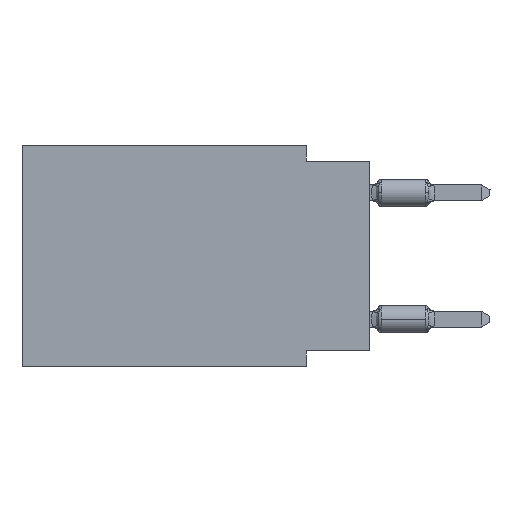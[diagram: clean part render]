
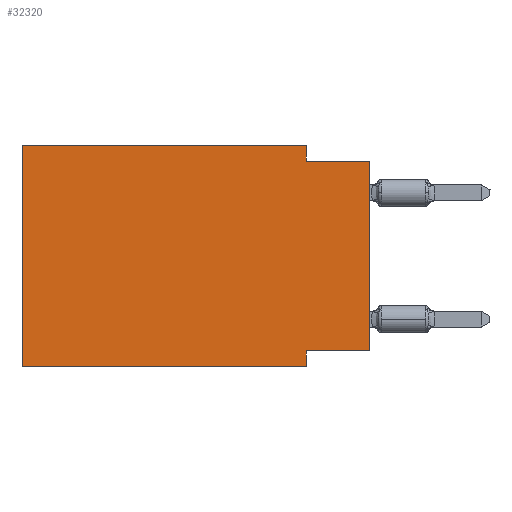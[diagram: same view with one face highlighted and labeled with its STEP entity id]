
A CAD part, left-side view. The second image highlights one B-rep face of the part: STEP entity #32320.
In plain terms, the highlighted planar face has unit normal (-1, 0, 0).
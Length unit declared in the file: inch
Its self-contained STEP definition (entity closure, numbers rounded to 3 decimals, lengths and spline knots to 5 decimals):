
#1415 = CARTESIAN_POINT ( 'NONE',  ( 0., 0., 0. ) ) ;
#2470 = ORIENTED_EDGE ( 'NONE', *, *, #6473, .T. ) ;
#2503 = DIRECTION ( 'NONE',  ( 0., 0., -1. ) ) ;
#2702 = VERTEX_POINT ( 'NONE', #35628 ) ;
#2811 = CARTESIAN_POINT ( 'NONE',  ( 0., 0.55, -0.35 ) ) ;
#3569 = DIRECTION ( 'NONE',  ( 0., 0., -1. ) ) ;
#3655 = CARTESIAN_POINT ( 'NONE',  ( 0., 0.55, 0. ) ) ;
#3764 = EDGE_LOOP ( 'NONE', ( #13858, #31833, #14776, #14707, #4587, #2470, #33046, #17247 ) ) ;
#4422 = VERTEX_POINT ( 'NONE', #27043 ) ;
#4587 = ORIENTED_EDGE ( 'NONE', *, *, #5260, .F. ) ;
#4892 = CARTESIAN_POINT ( 'NONE',  ( 0., 0., -0.325 ) ) ;
#5126 = EDGE_CURVE ( 'NONE', #27759, #5545, #11026, .T. ) ;
#5152 = PLANE ( 'NONE',  #29046 ) ;
#5260 = EDGE_CURVE ( 'NONE', #12288, #26938, #32330, .T. ) ;
#5545 = VERTEX_POINT ( 'NONE', #34624 ) ;
#5773 = EDGE_CURVE ( 'NONE', #4422, #5545, #32214, .T. ) ;
#5873 = EDGE_CURVE ( 'NONE', #35828, #36375, #8050, .T. ) ;
#6473 = EDGE_CURVE ( 'NONE', #12288, #36375, #16929, .T. ) ;
#6789 = DIRECTION ( 'NONE',  ( 0., 0., 1. ) ) ;
#7506 = CARTESIAN_POINT ( 'NONE',  ( 0., 0.1, -0.35 ) ) ;
#7661 = LINE ( 'NONE', #4892, #30694 ) ;
#8050 = LINE ( 'NONE', #7506, #25464 ) ;
#8244 = CARTESIAN_POINT ( 'NONE',  ( 0., 0., -0.025 ) ) ;
#9197 = DIRECTION ( 'NONE',  ( 1., 0., 0. ) ) ;
#9328 = DIRECTION ( 'NONE',  ( 0., 0., 1. ) ) ;
#11026 = LINE ( 'NONE', #8244, #29575 ) ;
#11267 = VECTOR ( 'NONE', #3569, 39.37008 ) ;
#12288 = VERTEX_POINT ( 'NONE', #17860 ) ;
#12664 = EDGE_CURVE ( 'NONE', #26938, #2702, #20746, .T. ) ;
#13858 = ORIENTED_EDGE ( 'NONE', *, *, #5773, .T. ) ;
#14700 = CARTESIAN_POINT ( 'NONE',  ( 0., 0.1, -0.025 ) ) ;
#14707 = ORIENTED_EDGE ( 'NONE', *, *, #12664, .F. ) ;
#14776 = ORIENTED_EDGE ( 'NONE', *, *, #27852, .F. ) ;
#15368 = VECTOR ( 'NONE', #9328, 39.37008 ) ;
#16929 = LINE ( 'NONE', #2811, #23554 ) ;
#17247 = ORIENTED_EDGE ( 'NONE', *, *, #19957, .F. ) ;
#17860 = CARTESIAN_POINT ( 'NONE',  ( 0., 0.55, -0.35 ) ) ;
#18509 = CARTESIAN_POINT ( 'NONE',  ( 0., 0.55, 0. ) ) ;
#19590 = DIRECTION ( 'NONE',  ( 0., -1., 0. ) ) ;
#19957 = EDGE_CURVE ( 'NONE', #4422, #35828, #7661, .T. ) ;
#20277 = DIRECTION ( 'NONE',  ( 0., -1., 0. ) ) ;
#20746 = LINE ( 'NONE', #18509, #34149 ) ;
#21679 = FACE_OUTER_BOUND ( 'NONE', #3764, .T. ) ;
#23110 = VECTOR ( 'NONE', #6789, 39.37008 ) ;
#23554 = VECTOR ( 'NONE', #20277, 39.37008 ) ;
#24732 = DIRECTION ( 'NONE',  ( 0., 1., 0. ) ) ;
#24857 = CARTESIAN_POINT ( 'NONE',  ( 0., 0.1, -0.35 ) ) ;
#25464 = VECTOR ( 'NONE', #2503, 39.37008 ) ;
#25748 = DIRECTION ( 'NONE',  ( 0., 0., -1. ) ) ;
#26938 = VERTEX_POINT ( 'NONE', #3655 ) ;
#27043 = CARTESIAN_POINT ( 'NONE',  ( 0., 0., -0.325 ) ) ;
#27060 = CARTESIAN_POINT ( 'NONE',  ( 0., 0.1, 0. ) ) ;
#27759 = VERTEX_POINT ( 'NONE', #14700 ) ;
#27852 = EDGE_CURVE ( 'NONE', #2702, #27759, #29158, .T. ) ;
#29046 = AXIS2_PLACEMENT_3D ( 'NONE', #33359, #9197, #25748 ) ;
#29158 = LINE ( 'NONE', #27060, #11267 ) ;
#29575 = VECTOR ( 'NONE', #19590, 39.37008 ) ;
#30694 = VECTOR ( 'NONE', #24732, 39.37008 ) ;
#31272 = CARTESIAN_POINT ( 'NONE',  ( 0., 0.1, -0.325 ) ) ;
#31833 = ORIENTED_EDGE ( 'NONE', *, *, #5126, .F. ) ;
#32214 = LINE ( 'NONE', #1415, #23110 ) ;
#32320 = ADVANCED_FACE ( 'NONE', ( #21679 ), #5152, .F. ) ;
#32330 = LINE ( 'NONE', #34748, #15368 ) ;
#32946 = DIRECTION ( 'NONE',  ( 0., -1., 0. ) ) ;
#33046 = ORIENTED_EDGE ( 'NONE', *, *, #5873, .F. ) ;
#33359 = CARTESIAN_POINT ( 'NONE',  ( 0., 0.55, 0. ) ) ;
#34149 = VECTOR ( 'NONE', #32946, 39.37008 ) ;
#34624 = CARTESIAN_POINT ( 'NONE',  ( 0., 0., -0.025 ) ) ;
#34748 = CARTESIAN_POINT ( 'NONE',  ( 0., 0.55, 0. ) ) ;
#35628 = CARTESIAN_POINT ( 'NONE',  ( 0., 0.1, 0. ) ) ;
#35828 = VERTEX_POINT ( 'NONE', #31272 ) ;
#36375 = VERTEX_POINT ( 'NONE', #24857 ) ;
